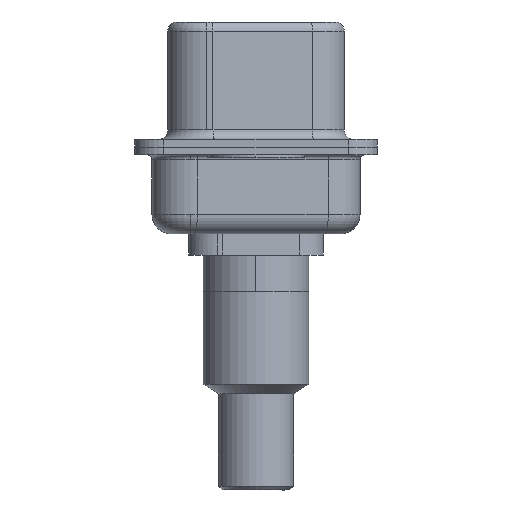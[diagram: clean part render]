
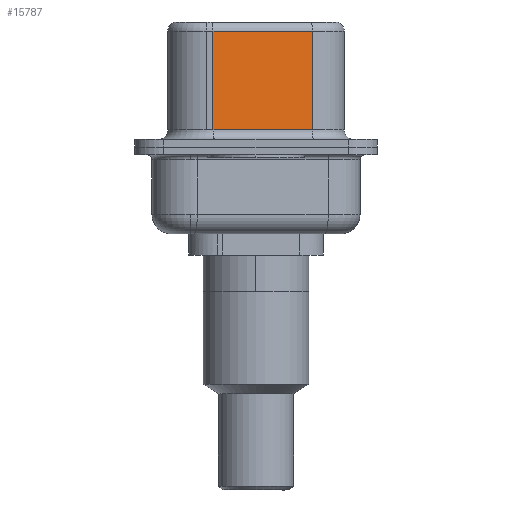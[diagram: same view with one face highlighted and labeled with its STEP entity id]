
A CAD part, left-side view. The second image highlights one B-rep face of the part: STEP entity #15787.
In plain terms, the highlighted planar face has unit normal (-0.985, -0.174, 0).
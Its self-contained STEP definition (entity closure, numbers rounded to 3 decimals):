
#964 = DIRECTION ( 'NONE',  ( 0., 0., -1. ) ) ;
#1255 = PLANE ( 'NONE',  #12060 ) ;
#1526 = DIRECTION ( 'NONE',  ( 0.985, 0.174, 0. ) ) ;
#1577 = CARTESIAN_POINT ( 'NONE',  ( 4.565, -2.927, 0.9 ) ) ;
#1629 = VERTEX_POINT ( 'NONE', #1577 ) ;
#1947 = VECTOR ( 'NONE', #964, 1000. ) ;
#3715 = FACE_OUTER_BOUND ( 'NONE', #11558, .T. ) ;
#3882 = EDGE_CURVE ( 'NONE', #8608, #1629, #17117, .T. ) ;
#4724 = EDGE_CURVE ( 'NONE', #5766, #1629, #11154, .T. ) ;
#5280 = LINE ( 'NONE', #13455, #1947 ) ;
#5766 = VERTEX_POINT ( 'NONE', #15046 ) ;
#5780 = ORIENTED_EDGE ( 'NONE', *, *, #6456, .T. ) ;
#5995 = EDGE_CURVE ( 'NONE', #15141, #5766, #5280, .T. ) ;
#6328 = CARTESIAN_POINT ( 'NONE',  ( 4.565, -2.927, 6.02 ) ) ;
#6456 = EDGE_CURVE ( 'NONE', #8608, #15141, #10117, .T. ) ;
#7408 = ORIENTED_EDGE ( 'NONE', *, *, #3882, .F. ) ;
#7561 = DIRECTION ( 'NONE',  ( 0.174, -0.985, 0. ) ) ;
#8608 = VERTEX_POINT ( 'NONE', #6328 ) ;
#8961 = CARTESIAN_POINT ( 'NONE',  ( 4.565, -2.927, 6.02 ) ) ;
#9253 = CARTESIAN_POINT ( 'NONE',  ( 4.565, -2.927, 6.52 ) ) ;
#9408 = VECTOR ( 'NONE', #9688, 1000. ) ;
#9679 = VECTOR ( 'NONE', #11870, 1000. ) ;
#9688 = DIRECTION ( 'NONE',  ( 0., 0., -1. ) ) ;
#10117 = LINE ( 'NONE', #8961, #9679 ) ;
#10498 = ORIENTED_EDGE ( 'NONE', *, *, #5995, .T. ) ;
#10686 = DIRECTION ( 'NONE',  ( -0.174, 0.985, 0. ) ) ;
#11154 = LINE ( 'NONE', #14346, #14664 ) ;
#11558 = EDGE_LOOP ( 'NONE', ( #7408, #5780, #10498, #14879 ) ) ;
#11727 = CARTESIAN_POINT ( 'NONE',  ( 3.655, 2.233, 6.02 ) ) ;
#11870 = DIRECTION ( 'NONE',  ( -0.174, 0.985, 0. ) ) ;
#12060 = AXIS2_PLACEMENT_3D ( 'NONE', #9253, #1526, #10686 ) ;
#13455 = CARTESIAN_POINT ( 'NONE',  ( 3.655, 2.233, 6.52 ) ) ;
#14346 = CARTESIAN_POINT ( 'NONE',  ( 4.565, -2.927, 0.9 ) ) ;
#14664 = VECTOR ( 'NONE', #7561, 1000. ) ;
#14879 = ORIENTED_EDGE ( 'NONE', *, *, #4724, .T. ) ;
#15046 = CARTESIAN_POINT ( 'NONE',  ( 3.655, 2.233, 0.9 ) ) ;
#15141 = VERTEX_POINT ( 'NONE', #11727 ) ;
#15787 = ADVANCED_FACE ( 'NONE', ( #3715 ), #1255, .F. ) ;
#16084 = CARTESIAN_POINT ( 'NONE',  ( 4.565, -2.927, 6.52 ) ) ;
#17117 = LINE ( 'NONE', #16084, #9408 ) ;
